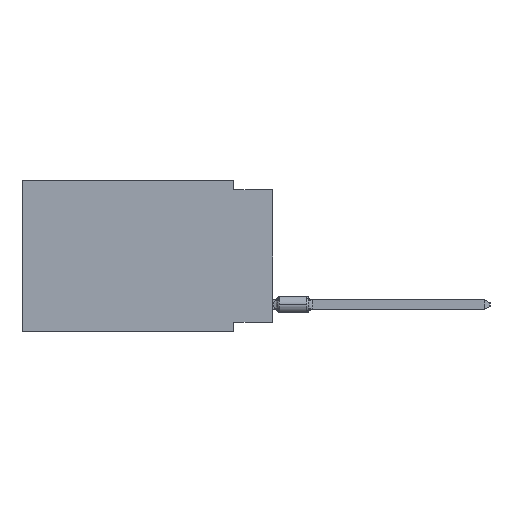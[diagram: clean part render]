
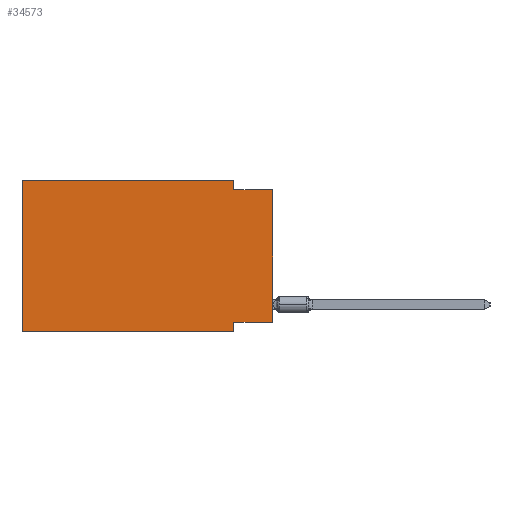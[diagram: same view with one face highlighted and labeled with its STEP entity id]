
A CAD part, left-side view. The second image highlights one B-rep face of the part: STEP entity #34573.
In plain terms, the highlighted planar face has unit normal (-1, 0, 0).
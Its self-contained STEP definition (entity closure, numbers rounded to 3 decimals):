
#172 = LINE ( 'NONE', #18669, #31896 ) ;
#593 = DIRECTION ( 'NONE',  ( 0., 0., 1. ) ) ;
#644 = LINE ( 'NONE', #33236, #20329 ) ;
#1098 = VECTOR ( 'NONE', #30973, 1000. ) ;
#1703 = ORIENTED_EDGE ( 'NONE', *, *, #30902, .T. ) ;
#2095 = VERTEX_POINT ( 'NONE', #19358 ) ;
#2282 = CARTESIAN_POINT ( 'NONE',  ( 0., 16.383, -9.906 ) ) ;
#2828 = VECTOR ( 'NONE', #28031, 1000. ) ;
#3572 = LINE ( 'NONE', #6021, #23777 ) ;
#3789 = EDGE_CURVE ( 'NONE', #20863, #31564, #32891, .T. ) ;
#6021 = CARTESIAN_POINT ( 'NONE',  ( 0., 0., 0. ) ) ;
#6760 = DIRECTION ( 'NONE',  ( 0., -1., 0. ) ) ;
#6878 = CARTESIAN_POINT ( 'NONE',  ( 0., 0., -9.271 ) ) ;
#7526 = CARTESIAN_POINT ( 'NONE',  ( 0., 2.54, -0.635 ) ) ;
#8477 = ORIENTED_EDGE ( 'NONE', *, *, #18156, .T. ) ;
#8502 = CARTESIAN_POINT ( 'NONE',  ( 0., 16.383, 0. ) ) ;
#9318 = LINE ( 'NONE', #33724, #2828 ) ;
#9502 = PLANE ( 'NONE',  #13530 ) ;
#10931 = EDGE_CURVE ( 'NONE', #31564, #17190, #30773, .T. ) ;
#11774 = DIRECTION ( 'NONE',  ( 0., 0., -1. ) ) ;
#13321 = VECTOR ( 'NONE', #30440, 1000. ) ;
#13530 = AXIS2_PLACEMENT_3D ( 'NONE', #18441, #21920, #37559 ) ;
#15020 = DIRECTION ( 'NONE',  ( 0., 1., 0. ) ) ;
#15431 = CARTESIAN_POINT ( 'NONE',  ( 0., 16.383, 0. ) ) ;
#15439 = VERTEX_POINT ( 'NONE', #2282 ) ;
#17031 = ORIENTED_EDGE ( 'NONE', *, *, #18216, .F. ) ;
#17190 = VERTEX_POINT ( 'NONE', #7526 ) ;
#17493 = EDGE_CURVE ( 'NONE', #21879, #35951, #172, .T. ) ;
#18156 = EDGE_CURVE ( 'NONE', #15439, #32942, #9318, .T. ) ;
#18216 = EDGE_CURVE ( 'NONE', #35951, #32942, #39605, .T. ) ;
#18441 = CARTESIAN_POINT ( 'NONE',  ( 0., 16.383, 0. ) ) ;
#18470 = ORIENTED_EDGE ( 'NONE', *, *, #3789, .F. ) ;
#18664 = CARTESIAN_POINT ( 'NONE',  ( 0., 2.54, -9.906 ) ) ;
#18669 = CARTESIAN_POINT ( 'NONE',  ( 0., 0., -9.271 ) ) ;
#19358 = CARTESIAN_POINT ( 'NONE',  ( 0., 0., -0.635 ) ) ;
#20181 = CARTESIAN_POINT ( 'NONE',  ( 0., 2.54, 0. ) ) ;
#20329 = VECTOR ( 'NONE', #6760, 1000. ) ;
#20863 = VERTEX_POINT ( 'NONE', #38953 ) ;
#21879 = VERTEX_POINT ( 'NONE', #6878 ) ;
#21881 = DIRECTION ( 'NONE',  ( 0., 0., 1. ) ) ;
#21920 = DIRECTION ( 'NONE',  ( 1., 0., 0. ) ) ;
#23777 = VECTOR ( 'NONE', #21881, 1000. ) ;
#24761 = ORIENTED_EDGE ( 'NONE', *, *, #17493, .F. ) ;
#27373 = CARTESIAN_POINT ( 'NONE',  ( 0., 2.54, -9.271 ) ) ;
#28031 = DIRECTION ( 'NONE',  ( 0., -1., 0. ) ) ;
#28411 = FACE_OUTER_BOUND ( 'NONE', #36704, .T. ) ;
#28833 = EDGE_CURVE ( 'NONE', #17190, #2095, #644, .T. ) ;
#30440 = DIRECTION ( 'NONE',  ( 0., -1., 0. ) ) ;
#30745 = VECTOR ( 'NONE', #11774, 1000. ) ;
#30773 = LINE ( 'NONE', #34224, #1098 ) ;
#30885 = LINE ( 'NONE', #15431, #32287 ) ;
#30902 = EDGE_CURVE ( 'NONE', #21879, #2095, #3572, .T. ) ;
#30973 = DIRECTION ( 'NONE',  ( 0., 0., -1. ) ) ;
#31564 = VERTEX_POINT ( 'NONE', #20181 ) ;
#31893 = EDGE_CURVE ( 'NONE', #15439, #20863, #30885, .T. ) ;
#31896 = VECTOR ( 'NONE', #15020, 1000. ) ;
#32152 = ORIENTED_EDGE ( 'NONE', *, *, #31893, .F. ) ;
#32287 = VECTOR ( 'NONE', #593, 1000. ) ;
#32891 = LINE ( 'NONE', #8502, #13321 ) ;
#32942 = VERTEX_POINT ( 'NONE', #39239 ) ;
#33236 = CARTESIAN_POINT ( 'NONE',  ( 0., 0., -0.635 ) ) ;
#33724 = CARTESIAN_POINT ( 'NONE',  ( 0., 16.383, -9.906 ) ) ;
#34224 = CARTESIAN_POINT ( 'NONE',  ( 0., 2.54, 0. ) ) ;
#34573 = ADVANCED_FACE ( 'NONE', ( #28411 ), #9502, .F. ) ;
#35951 = VERTEX_POINT ( 'NONE', #27373 ) ;
#36167 = ORIENTED_EDGE ( 'NONE', *, *, #10931, .F. ) ;
#36704 = EDGE_LOOP ( 'NONE', ( #1703, #38183, #36167, #18470, #32152, #8477, #17031, #24761 ) ) ;
#37559 = DIRECTION ( 'NONE',  ( 0., 0., -1. ) ) ;
#38183 = ORIENTED_EDGE ( 'NONE', *, *, #28833, .F. ) ;
#38953 = CARTESIAN_POINT ( 'NONE',  ( 0., 16.383, 0. ) ) ;
#39239 = CARTESIAN_POINT ( 'NONE',  ( 0., 2.54, -9.906 ) ) ;
#39605 = LINE ( 'NONE', #18664, #30745 ) ;
